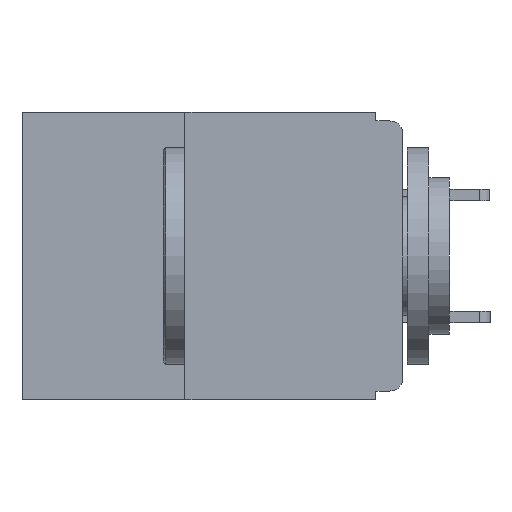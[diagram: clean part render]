
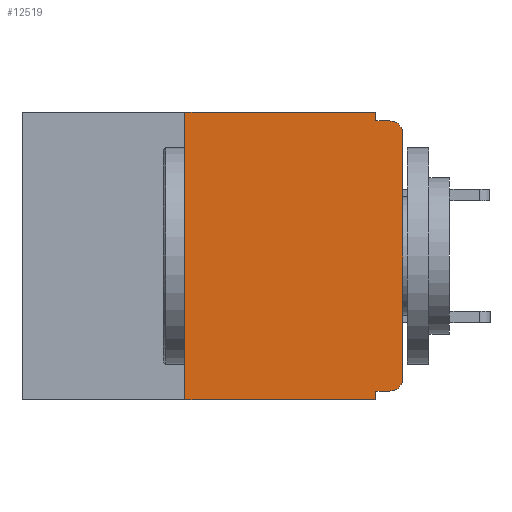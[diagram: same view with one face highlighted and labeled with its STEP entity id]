
A CAD part, left-side view. The second image highlights one B-rep face of the part: STEP entity #12519.
In plain terms, the highlighted planar face has unit normal (-1, 0, 0).
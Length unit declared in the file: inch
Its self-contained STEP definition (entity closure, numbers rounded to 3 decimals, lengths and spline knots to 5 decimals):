
#39 = CARTESIAN_POINT ( 'NONE',  ( 0., 0., -0.01 ) ) ;
#338 = VERTEX_POINT ( 'NONE', #16550 ) ;
#791 = CARTESIAN_POINT ( 'NONE',  ( 0., 0.015, -0.32 ) ) ;
#955 = VECTOR ( 'NONE', #2444, 39.37008 ) ;
#1465 = ORIENTED_EDGE ( 'NONE', *, *, #11535, .T. ) ;
#1992 = EDGE_CURVE ( 'NONE', #3344, #10032, #13638, .T. ) ;
#2004 = LINE ( 'NONE', #39, #2511 ) ;
#2188 = VERTEX_POINT ( 'NONE', #791 ) ;
#2405 = PLANE ( 'NONE',  #16981 ) ;
#2444 = DIRECTION ( 'NONE',  ( 0., 0., -1. ) ) ;
#2511 = VECTOR ( 'NONE', #13927, 39.37008 ) ;
#3078 = EDGE_CURVE ( 'NONE', #3344, #19187, #3318, .T. ) ;
#3126 = ORIENTED_EDGE ( 'NONE', *, *, #13862, .F. ) ;
#3275 = EDGE_LOOP ( 'NONE', ( #1465, #4252, #5732, #18605, #14431, #11434, #7533, #6582, #3126, #4521 ) ) ;
#3318 = LINE ( 'NONE', #11248, #14503 ) ;
#3344 = VERTEX_POINT ( 'NONE', #19076 ) ;
#3566 = VECTOR ( 'NONE', #10359, 39.37008 ) ;
#3927 = CARTESIAN_POINT ( 'NONE',  ( 0., 0.031, 0. ) ) ;
#4252 = ORIENTED_EDGE ( 'NONE', *, *, #9908, .T. ) ;
#4284 = VECTOR ( 'NONE', #16516, 39.37008 ) ;
#4309 = EDGE_CURVE ( 'NONE', #14987, #11884, #2004, .T. ) ;
#4521 = ORIENTED_EDGE ( 'NONE', *, *, #6871, .T. ) ;
#4601 = VECTOR ( 'NONE', #13570, 39.37008 ) ;
#5409 = CARTESIAN_POINT ( 'NONE',  ( 0., 0.031, -0.32 ) ) ;
#5456 = DIRECTION ( 'NONE',  ( 0., 0., -1. ) ) ;
#5470 = DIRECTION ( 'NONE',  ( -1., 0., 0. ) ) ;
#5489 = CARTESIAN_POINT ( 'NONE',  ( 0., 0.015, -0.305 ) ) ;
#5666 = DIRECTION ( 'NONE',  ( 0., 0., -1. ) ) ;
#5732 = ORIENTED_EDGE ( 'NONE', *, *, #4309, .F. ) ;
#6355 = EDGE_CURVE ( 'NONE', #16607, #14987, #16679, .T. ) ;
#6582 = ORIENTED_EDGE ( 'NONE', *, *, #19444, .F. ) ;
#6871 = EDGE_CURVE ( 'NONE', #2188, #8948, #18653, .T. ) ;
#7059 = DIRECTION ( 'NONE',  ( 0., -1., 0. ) ) ;
#7533 = ORIENTED_EDGE ( 'NONE', *, *, #1992, .T. ) ;
#7747 = CARTESIAN_POINT ( 'NONE',  ( 0., 0., -0.32 ) ) ;
#8201 = AXIS2_PLACEMENT_3D ( 'NONE', #5489, #5470, #5456 ) ;
#8303 = CARTESIAN_POINT ( 'NONE',  ( 0., 0.031, 0. ) ) ;
#8624 = CARTESIAN_POINT ( 'NONE',  ( 0., 0., -0.305 ) ) ;
#8852 = CARTESIAN_POINT ( 'NONE',  ( 0., 0.031, -0.33 ) ) ;
#8948 = VERTEX_POINT ( 'NONE', #8624 ) ;
#9908 = EDGE_CURVE ( 'NONE', #338, #11884, #16065, .T. ) ;
#10032 = VERTEX_POINT ( 'NONE', #8852 ) ;
#10317 = DIRECTION ( 'NONE',  ( 0., 0., -1. ) ) ;
#10321 = DIRECTION ( 'NONE',  ( -1., 0., 0. ) ) ;
#10348 = CARTESIAN_POINT ( 'NONE',  ( 0., 0.015, -0.025 ) ) ;
#10359 = DIRECTION ( 'NONE',  ( 0., 0., -1. ) ) ;
#10940 = CARTESIAN_POINT ( 'NONE',  ( 0., 0., 0. ) ) ;
#10941 = LINE ( 'NONE', #13020, #14378 ) ;
#11248 = CARTESIAN_POINT ( 'NONE',  ( 0., 0.25, -0.33 ) ) ;
#11274 = DIRECTION ( 'NONE',  ( 0., 0., 1. ) ) ;
#11300 = VECTOR ( 'NONE', #19555, 39.37008 ) ;
#11434 = ORIENTED_EDGE ( 'NONE', *, *, #3078, .F. ) ;
#11535 = EDGE_CURVE ( 'NONE', #8948, #338, #15588, .T. ) ;
#11884 = VERTEX_POINT ( 'NONE', #17440 ) ;
#12447 = LINE ( 'NONE', #7747, #4284 ) ;
#12519 = ADVANCED_FACE ( 'NONE', ( #17386 ), #2405, .F. ) ;
#13020 = CARTESIAN_POINT ( 'NONE',  ( 0., 0.437, 0. ) ) ;
#13188 = CARTESIAN_POINT ( 'NONE',  ( 0., 0.437, 0. ) ) ;
#13336 = CARTESIAN_POINT ( 'NONE',  ( 0., 0.031, -0.33 ) ) ;
#13570 = DIRECTION ( 'NONE',  ( 0., -1., 0. ) ) ;
#13638 = LINE ( 'NONE', #17490, #4601 ) ;
#13862 = EDGE_CURVE ( 'NONE', #2188, #19034, #12447, .T. ) ;
#13927 = DIRECTION ( 'NONE',  ( 0., -1., 0. ) ) ;
#14378 = VECTOR ( 'NONE', #7059, 39.37008 ) ;
#14431 = ORIENTED_EDGE ( 'NONE', *, *, #15992, .F. ) ;
#14503 = VECTOR ( 'NONE', #11274, 39.37008 ) ;
#14612 = DIRECTION ( 'NONE',  ( 1., 0., 0. ) ) ;
#14987 = VERTEX_POINT ( 'NONE', #17723 ) ;
#15556 = CARTESIAN_POINT ( 'NONE',  ( 0., 0.25, 0. ) ) ;
#15588 = LINE ( 'NONE', #10940, #11300 ) ;
#15597 = LINE ( 'NONE', #13336, #3566 ) ;
#15992 = EDGE_CURVE ( 'NONE', #19187, #16607, #10941, .T. ) ;
#16065 = CIRCLE ( 'NONE', #19201, 0.015 ) ;
#16516 = DIRECTION ( 'NONE',  ( 0., 1., 0. ) ) ;
#16550 = CARTESIAN_POINT ( 'NONE',  ( 0., 0., -0.025 ) ) ;
#16607 = VERTEX_POINT ( 'NONE', #3927 ) ;
#16679 = LINE ( 'NONE', #8303, #955 ) ;
#16981 = AXIS2_PLACEMENT_3D ( 'NONE', #13188, #14612, #5666 ) ;
#17386 = FACE_OUTER_BOUND ( 'NONE', #3275, .T. ) ;
#17440 = CARTESIAN_POINT ( 'NONE',  ( 0., 0.015, -0.01 ) ) ;
#17490 = CARTESIAN_POINT ( 'NONE',  ( 0., 0.437, -0.33 ) ) ;
#17723 = CARTESIAN_POINT ( 'NONE',  ( 0., 0.031, -0.01 ) ) ;
#18605 = ORIENTED_EDGE ( 'NONE', *, *, #6355, .F. ) ;
#18653 = CIRCLE ( 'NONE', #8201, 0.015 ) ;
#19034 = VERTEX_POINT ( 'NONE', #5409 ) ;
#19076 = CARTESIAN_POINT ( 'NONE',  ( 0., 0.25, -0.33 ) ) ;
#19187 = VERTEX_POINT ( 'NONE', #15556 ) ;
#19201 = AXIS2_PLACEMENT_3D ( 'NONE', #10348, #10321, #10317 ) ;
#19444 = EDGE_CURVE ( 'NONE', #19034, #10032, #15597, .T. ) ;
#19555 = DIRECTION ( 'NONE',  ( 0., 0., 1. ) ) ;
